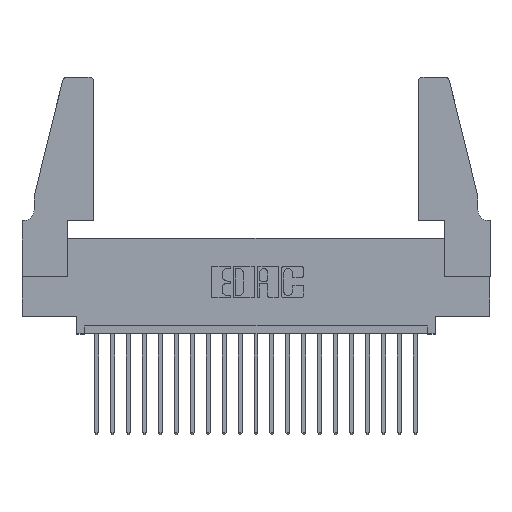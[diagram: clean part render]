
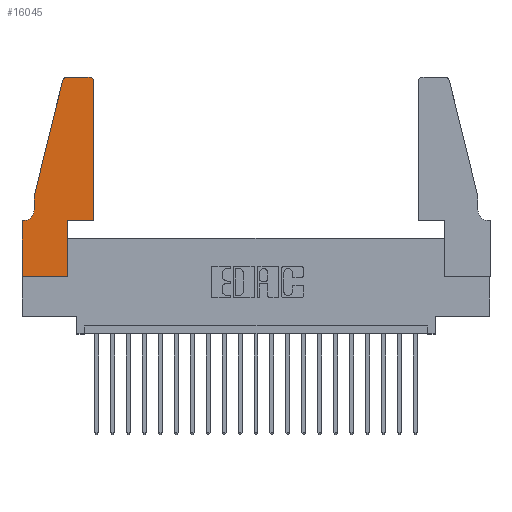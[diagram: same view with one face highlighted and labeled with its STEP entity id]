
A CAD part, top view. The second image highlights one B-rep face of the part: STEP entity #16045.
In plain terms, the highlighted planar face has unit normal (0, 0, 1).
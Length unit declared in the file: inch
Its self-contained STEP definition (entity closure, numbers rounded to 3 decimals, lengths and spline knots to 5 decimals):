
#25 = CARTESIAN_POINT ( 'NONE',  ( 0.0755, 0.42, 0.37 ) ) ;
#292 = DIRECTION ( 'NONE',  ( 1., 0., 0. ) ) ;
#556 = VECTOR ( 'NONE', #19261, 39.37008 ) ;
#1159 = EDGE_CURVE ( 'NONE', #18400, #19728, #3909, .T. ) ;
#1371 = EDGE_CURVE ( 'NONE', #4190, #4789, #11006, .T. ) ;
#1594 = CARTESIAN_POINT ( 'NONE',  ( 0.0755, 0.5, 0.37 ) ) ;
#1770 = CARTESIAN_POINT ( 'NONE',  ( 0.2865, 0.35, 0.37 ) ) ;
#1979 = EDGE_CURVE ( 'NONE', #12712, #17555, #14516, .T. ) ;
#2632 = ORIENTED_EDGE ( 'NONE', *, *, #12999, .T. ) ;
#2690 = AXIS2_PLACEMENT_3D ( 'NONE', #19741, #13267, #292 ) ;
#2872 = CARTESIAN_POINT ( 'NONE',  ( 0.4505, 0.35, 0.37 ) ) ;
#2873 = CARTESIAN_POINT ( 'NONE',  ( 0.4205, 1.22, 0.37 ) ) ;
#3424 = CARTESIAN_POINT ( 'NONE',  ( 0.0055, 0.42, 0.37 ) ) ;
#3738 = CARTESIAN_POINT ( 'NONE',  ( 0.284, 1.25, 0.37 ) ) ;
#3863 = CARTESIAN_POINT ( 'NONE',  ( 0.0055, 0.35, 0.37 ) ) ;
#3909 = LINE ( 'NONE', #2872, #20312 ) ;
#3937 = DIRECTION ( 'NONE',  ( -1., 0., 0. ) ) ;
#4190 = VERTEX_POINT ( 'NONE', #25 ) ;
#4489 = CIRCLE ( 'NONE', #7669, 0.03 ) ;
#4555 = CARTESIAN_POINT ( 'NONE',  ( 0.0755, 0.5, 0.37 ) ) ;
#4632 = DIRECTION ( 'NONE',  ( 0., 1., 0. ) ) ;
#4685 = DIRECTION ( 'NONE',  ( 0., -1., 0. ) ) ;
#4789 = VERTEX_POINT ( 'NONE', #3863 ) ;
#4799 = DIRECTION ( 'NONE',  ( 0., 1., 0. ) ) ;
#5135 = ORIENTED_EDGE ( 'NONE', *, *, #18628, .T. ) ;
#5312 = CARTESIAN_POINT ( 'NONE',  ( 0.2865, 0.35, 0.37 ) ) ;
#5918 = EDGE_CURVE ( 'NONE', #17555, #8703, #12259, .T. ) ;
#6657 = DIRECTION ( 'NONE',  ( -1., 0., 0. ) ) ;
#6730 = AXIS2_PLACEMENT_3D ( 'NONE', #3424, #19466, #6657 ) ;
#7070 = VERTEX_POINT ( 'NONE', #11566 ) ;
#7306 = LINE ( 'NONE', #20766, #19696 ) ;
#7307 = CARTESIAN_POINT ( 'NONE',  ( 0., 0., 0.37 ) ) ;
#7367 = DIRECTION ( 'NONE',  ( 1., 0., 0. ) ) ;
#7393 = PLANE ( 'NONE',  #17446 ) ;
#7571 = FACE_OUTER_BOUND ( 'NONE', #16125, .T. ) ;
#7669 = AXIS2_PLACEMENT_3D ( 'NONE', #2873, #17463, #7764 ) ;
#7764 = DIRECTION ( 'NONE',  ( 1., 0., 0. ) ) ;
#7798 = LINE ( 'NONE', #12638, #8823 ) ;
#8471 = DIRECTION ( 'NONE',  ( 0., -1., 0. ) ) ;
#8600 = CARTESIAN_POINT ( 'NONE',  ( 0., 0.35, 0.37 ) ) ;
#8703 = VERTEX_POINT ( 'NONE', #12980 ) ;
#8729 = ORIENTED_EDGE ( 'NONE', *, *, #1371, .T. ) ;
#8823 = VECTOR ( 'NONE', #17859, 39.37008 ) ;
#9091 = ORIENTED_EDGE ( 'NONE', *, *, #5918, .T. ) ;
#9168 = EDGE_CURVE ( 'NONE', #17124, #17732, #9828, .T. ) ;
#9398 = VECTOR ( 'NONE', #8471, 39.37008 ) ;
#9400 = DIRECTION ( 'NONE',  ( 0., 0., 1. ) ) ;
#9473 = VERTEX_POINT ( 'NONE', #17637 ) ;
#9828 = LINE ( 'NONE', #1770, #13381 ) ;
#10047 = ORIENTED_EDGE ( 'NONE', *, *, #10599, .T. ) ;
#10599 = EDGE_CURVE ( 'NONE', #7070, #12712, #7798, .T. ) ;
#10873 = CARTESIAN_POINT ( 'NONE',  ( 0.25487, 1.22718, 0.37 ) ) ;
#11006 = CIRCLE ( 'NONE', #6730, 0.07 ) ;
#11507 = ORIENTED_EDGE ( 'NONE', *, *, #18049, .T. ) ;
#11566 = CARTESIAN_POINT ( 'NONE',  ( 0.4205, 1.25, 0.37 ) ) ;
#12129 = ORIENTED_EDGE ( 'NONE', *, *, #1979, .T. ) ;
#12259 = LINE ( 'NONE', #1594, #556 ) ;
#12580 = CARTESIAN_POINT ( 'NONE',  ( 0.0755, 0.35, 0.37 ) ) ;
#12638 = CARTESIAN_POINT ( 'NONE',  ( 0.2605, 1.25, 0.37 ) ) ;
#12668 = VECTOR ( 'NONE', #3937, 39.37008 ) ;
#12711 = DIRECTION ( 'NONE',  ( 1., 0., 0. ) ) ;
#12712 = VERTEX_POINT ( 'NONE', #3738 ) ;
#12900 = ORIENTED_EDGE ( 'NONE', *, *, #16099, .T. ) ;
#12980 = CARTESIAN_POINT ( 'NONE',  ( 0.0755, 0.5, 0.37 ) ) ;
#12999 = EDGE_CURVE ( 'NONE', #9473, #17124, #20291, .T. ) ;
#13267 = DIRECTION ( 'NONE',  ( 0., 0., 1. ) ) ;
#13381 = VECTOR ( 'NONE', #4632, 39.37008 ) ;
#13470 = VECTOR ( 'NONE', #4685, 39.37008 ) ;
#13914 = CARTESIAN_POINT ( 'NONE',  ( 0., 0.35, 0.37 ) ) ;
#14516 = CIRCLE ( 'NONE', #2690, 0.03 ) ;
#14593 = ORIENTED_EDGE ( 'NONE', *, *, #9168, .T. ) ;
#14886 = ORIENTED_EDGE ( 'NONE', *, *, #1159, .T. ) ;
#15126 = ORIENTED_EDGE ( 'NONE', *, *, #19100, .T. ) ;
#15217 = ORIENTED_EDGE ( 'NONE', *, *, #17132, .T. ) ;
#15766 = LINE ( 'NONE', #18154, #9398 ) ;
#16021 = LINE ( 'NONE', #4555, #13470 ) ;
#16045 = ADVANCED_FACE ( 'NONE', ( #7571 ), #7393, .T. ) ;
#16099 = EDGE_CURVE ( 'NONE', #19728, #7070, #4489, .T. ) ;
#16125 = EDGE_LOOP ( 'NONE', ( #10047, #12129, #9091, #15217, #8729, #5135, #11507, #2632, #14593, #15126, #14886, #12900 ) ) ;
#16481 = LINE ( 'NONE', #12580, #12668 ) ;
#17124 = VERTEX_POINT ( 'NONE', #19999 ) ;
#17132 = EDGE_CURVE ( 'NONE', #8703, #4190, #16021, .T. ) ;
#17446 = AXIS2_PLACEMENT_3D ( 'NONE', #13914, #9400, #12711 ) ;
#17463 = DIRECTION ( 'NONE',  ( 0., 0., 1. ) ) ;
#17555 = VERTEX_POINT ( 'NONE', #10873 ) ;
#17637 = CARTESIAN_POINT ( 'NONE',  ( 0., 0., 0.37 ) ) ;
#17732 = VERTEX_POINT ( 'NONE', #5312 ) ;
#17804 = VECTOR ( 'NONE', #7367, 39.37008 ) ;
#17859 = DIRECTION ( 'NONE',  ( -1., 0., 0. ) ) ;
#18049 = EDGE_CURVE ( 'NONE', #20346, #9473, #15766, .T. ) ;
#18154 = CARTESIAN_POINT ( 'NONE',  ( 0., 0., 0.37 ) ) ;
#18400 = VERTEX_POINT ( 'NONE', #20587 ) ;
#18628 = EDGE_CURVE ( 'NONE', #4789, #20346, #16481, .T. ) ;
#19100 = EDGE_CURVE ( 'NONE', #17732, #18400, #7306, .T. ) ;
#19261 = DIRECTION ( 'NONE',  ( -0.239, -0.971, 0. ) ) ;
#19466 = DIRECTION ( 'NONE',  ( 0., 0., -1. ) ) ;
#19696 = VECTOR ( 'NONE', #20557, 39.37008 ) ;
#19700 = CARTESIAN_POINT ( 'NONE',  ( 0.4505, 1.22, 0.37 ) ) ;
#19728 = VERTEX_POINT ( 'NONE', #19700 ) ;
#19741 = CARTESIAN_POINT ( 'NONE',  ( 0.284, 1.22, 0.37 ) ) ;
#19999 = CARTESIAN_POINT ( 'NONE',  ( 0.2865, 0., 0.37 ) ) ;
#20291 = LINE ( 'NONE', #7307, #17804 ) ;
#20312 = VECTOR ( 'NONE', #4799, 39.37008 ) ;
#20346 = VERTEX_POINT ( 'NONE', #8600 ) ;
#20557 = DIRECTION ( 'NONE',  ( 1., 0., 0. ) ) ;
#20587 = CARTESIAN_POINT ( 'NONE',  ( 0.4505, 0.35, 0.37 ) ) ;
#20766 = CARTESIAN_POINT ( 'NONE',  ( 0.4505, 0.35, 0.37 ) ) ;
